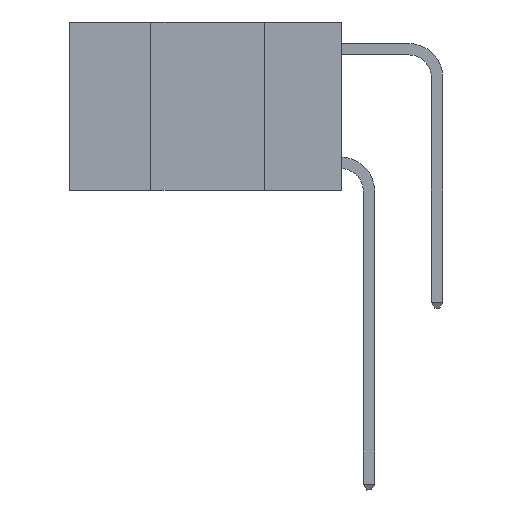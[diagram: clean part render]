
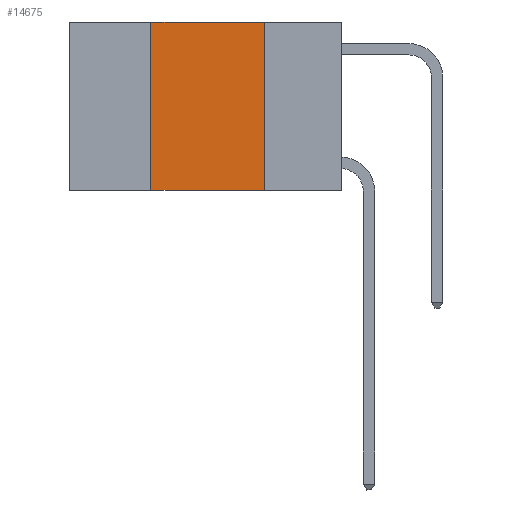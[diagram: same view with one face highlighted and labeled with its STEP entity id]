
A CAD part, left-side view. The second image highlights one B-rep face of the part: STEP entity #14675.
In plain terms, the highlighted planar face has unit normal (-1, 0, 0).
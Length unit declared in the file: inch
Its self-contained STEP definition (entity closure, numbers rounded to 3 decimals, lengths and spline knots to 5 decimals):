
#39 = DIRECTION ( 'NONE',  ( 0., 0., 1. ) ) ;
#208 = VERTEX_POINT ( 'NONE', #1398 ) ;
#1398 = CARTESIAN_POINT ( 'NONE',  ( 0., 0.42, -0.37 ) ) ;
#2122 = LINE ( 'NONE', #19177, #7391 ) ;
#3138 = EDGE_CURVE ( 'NONE', #208, #17280, #2122, .T. ) ;
#3278 = VECTOR ( 'NONE', #17683, 39.37008 ) ;
#4655 = CARTESIAN_POINT ( 'NONE',  ( 0., 0.17, -0.37 ) ) ;
#4862 = AXIS2_PLACEMENT_3D ( 'NONE', #18856, #17433, #14278 ) ;
#4943 = ORIENTED_EDGE ( 'NONE', *, *, #16282, .F. ) ;
#6748 = LINE ( 'NONE', #12894, #3278 ) ;
#7391 = VECTOR ( 'NONE', #11471, 39.37008 ) ;
#7833 = FACE_OUTER_BOUND ( 'NONE', #17631, .T. ) ;
#8030 = EDGE_CURVE ( 'NONE', #17696, #17280, #6748, .T. ) ;
#8431 = DIRECTION ( 'NONE',  ( 0., -1., 0. ) ) ;
#8537 = LINE ( 'NONE', #12976, #14920 ) ;
#9475 = ORIENTED_EDGE ( 'NONE', *, *, #8030, .F. ) ;
#11471 = DIRECTION ( 'NONE',  ( 0., -1., 0. ) ) ;
#12661 = PLANE ( 'NONE',  #4862 ) ;
#12894 = CARTESIAN_POINT ( 'NONE',  ( 0., 0.17, 0. ) ) ;
#12976 = CARTESIAN_POINT ( 'NONE',  ( 0., 0.6, 0. ) ) ;
#13262 = CARTESIAN_POINT ( 'NONE',  ( 0., 0.42, 0. ) ) ;
#13833 = LINE ( 'NONE', #16801, #15767 ) ;
#14278 = DIRECTION ( 'NONE',  ( 0., 0., -1. ) ) ;
#14675 = ADVANCED_FACE ( 'NONE', ( #7833 ), #12661, .F. ) ;
#14729 = VERTEX_POINT ( 'NONE', #13262 ) ;
#14920 = VECTOR ( 'NONE', #8431, 39.37008 ) ;
#15767 = VECTOR ( 'NONE', #39, 39.37008 ) ;
#15994 = ORIENTED_EDGE ( 'NONE', *, *, #19616, .F. ) ;
#16282 = EDGE_CURVE ( 'NONE', #14729, #17696, #8537, .T. ) ;
#16801 = CARTESIAN_POINT ( 'NONE',  ( 0., 0.42, 0. ) ) ;
#17280 = VERTEX_POINT ( 'NONE', #4655 ) ;
#17433 = DIRECTION ( 'NONE',  ( 1., 0., 0. ) ) ;
#17631 = EDGE_LOOP ( 'NONE', ( #9475, #4943, #15994, #19615 ) ) ;
#17683 = DIRECTION ( 'NONE',  ( 0., 0., -1. ) ) ;
#17696 = VERTEX_POINT ( 'NONE', #18465 ) ;
#18465 = CARTESIAN_POINT ( 'NONE',  ( 0., 0.17, 0. ) ) ;
#18856 = CARTESIAN_POINT ( 'NONE',  ( 0., 0.6, 0. ) ) ;
#19177 = CARTESIAN_POINT ( 'NONE',  ( 0., 0.6, -0.37 ) ) ;
#19615 = ORIENTED_EDGE ( 'NONE', *, *, #3138, .T. ) ;
#19616 = EDGE_CURVE ( 'NONE', #208, #14729, #13833, .T. ) ;
